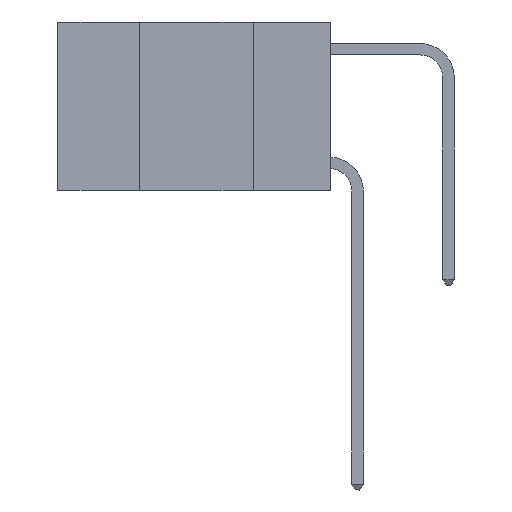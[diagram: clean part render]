
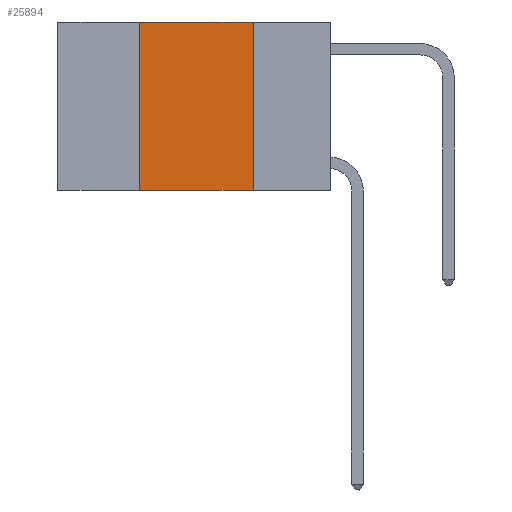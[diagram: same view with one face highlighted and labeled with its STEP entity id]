
A CAD part, left-side view. The second image highlights one B-rep face of the part: STEP entity #25894.
In plain terms, the highlighted planar face has unit normal (-1, 0, 0).
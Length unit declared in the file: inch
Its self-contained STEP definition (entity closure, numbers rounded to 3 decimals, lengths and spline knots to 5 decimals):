
#1705 = VERTEX_POINT ( 'NONE', #26562 ) ;
#2354 = DIRECTION ( 'NONE',  ( 0., 0., -1. ) ) ;
#3823 = VECTOR ( 'NONE', #9114, 39.37008 ) ;
#3865 = VECTOR ( 'NONE', #2354, 39.37008 ) ;
#4514 = LINE ( 'NONE', #15390, #22295 ) ;
#5113 = EDGE_CURVE ( 'NONE', #19874, #1705, #4514, .T. ) ;
#5542 = CARTESIAN_POINT ( 'NONE',  ( 0., 0.17, 0. ) ) ;
#7494 = VERTEX_POINT ( 'NONE', #25097 ) ;
#8795 = DIRECTION ( 'NONE',  ( 0., 0., -1. ) ) ;
#8971 = CARTESIAN_POINT ( 'NONE',  ( 0., 0.17, 0. ) ) ;
#9114 = DIRECTION ( 'NONE',  ( 0., -1., 0. ) ) ;
#13360 = LINE ( 'NONE', #18171, #3823 ) ;
#15390 = CARTESIAN_POINT ( 'NONE',  ( 0., 0.42, 0. ) ) ;
#15496 = CARTESIAN_POINT ( 'NONE',  ( 0., 0.42, -0.37 ) ) ;
#18126 = ORIENTED_EDGE ( 'NONE', *, *, #19988, .F. ) ;
#18146 = DIRECTION ( 'NONE',  ( 1., 0., 0. ) ) ;
#18171 = CARTESIAN_POINT ( 'NONE',  ( 0., 0.6, -0.37 ) ) ;
#19372 = LINE ( 'NONE', #28575, #28131 ) ;
#19665 = DIRECTION ( 'NONE',  ( 0., -1., 0. ) ) ;
#19874 = VERTEX_POINT ( 'NONE', #15496 ) ;
#19988 = EDGE_CURVE ( 'NONE', #23960, #7494, #29646, .T. ) ;
#20490 = DIRECTION ( 'NONE',  ( 0., 0., 1. ) ) ;
#20553 = CARTESIAN_POINT ( 'NONE',  ( 0., 0.6, 0. ) ) ;
#21290 = EDGE_LOOP ( 'NONE', ( #18126, #25314, #26900, #21542 ) ) ;
#21542 = ORIENTED_EDGE ( 'NONE', *, *, #28428, .T. ) ;
#22295 = VECTOR ( 'NONE', #20490, 39.37008 ) ;
#22962 = PLANE ( 'NONE',  #26224 ) ;
#23960 = VERTEX_POINT ( 'NONE', #5542 ) ;
#24353 = EDGE_CURVE ( 'NONE', #1705, #23960, #19372, .T. ) ;
#25097 = CARTESIAN_POINT ( 'NONE',  ( 0., 0.17, -0.37 ) ) ;
#25314 = ORIENTED_EDGE ( 'NONE', *, *, #24353, .F. ) ;
#25894 = ADVANCED_FACE ( 'NONE', ( #27211 ), #22962, .F. ) ;
#26224 = AXIS2_PLACEMENT_3D ( 'NONE', #20553, #18146, #8795 ) ;
#26562 = CARTESIAN_POINT ( 'NONE',  ( 0., 0.42, 0. ) ) ;
#26900 = ORIENTED_EDGE ( 'NONE', *, *, #5113, .F. ) ;
#27211 = FACE_OUTER_BOUND ( 'NONE', #21290, .T. ) ;
#28131 = VECTOR ( 'NONE', #19665, 39.37008 ) ;
#28428 = EDGE_CURVE ( 'NONE', #19874, #7494, #13360, .T. ) ;
#28575 = CARTESIAN_POINT ( 'NONE',  ( 0., 0.6, 0. ) ) ;
#29646 = LINE ( 'NONE', #8971, #3865 ) ;
